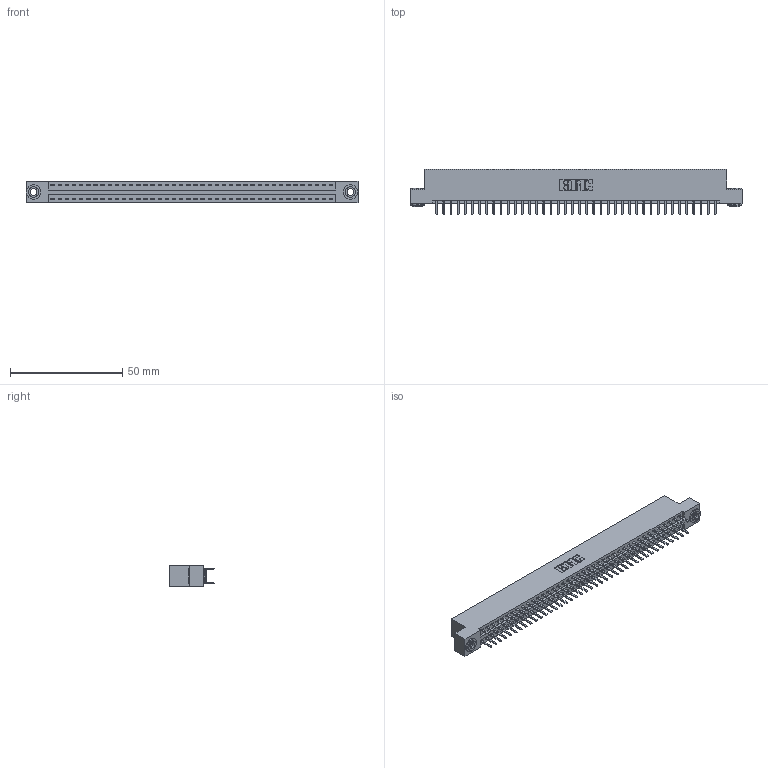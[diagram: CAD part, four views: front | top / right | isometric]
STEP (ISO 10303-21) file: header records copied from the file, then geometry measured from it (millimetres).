
FILE_DESCRIPTION (( 'STEP AP203' ), '1' );
FILE_NAME ('396-080-520-203.STEP', '2019-10-30T22:28:11', ( '' ), ( '' ), 'SwSTEP 2.0', 'SolidWorks 2016', '' );
FILE_SCHEMA (( 'CONFIG_CONTROL_DESIGN' ));
Length unit declared in the file: inch
Products named in the file (4): 396-080-520-203; 345-292-001_345-293-120; 345-250-002_345-250-002-102; 346 Part_Flush Mounting Lugs - 0.156 Dia-TH
Assembly tree (83 placements, depth 2):
  396-080-520-203
    346 Part_Flush Mounting Lugs - 0.156 Dia-TH
    345-292-001_345-293-120  x80
    345-250-002_345-250-002-102  x2
Bounding box: 147.57 x 20.02 x 9.4 mm (x, y, z)
Volume: 14359 mm3; surface area: 19837.7 mm2
Topology: 83 solids, 83 shells, 4640 faces, 13445 edges, 8746 vertices
Faces by surface type: plane 3046, cylinder 1586, cone 8
Entity records: 27138 total; most frequent: CARTESIAN_POINT 4463, ORIENTED_EDGE 4378, DIRECTION 4003, EDGE_CURVE 2189, VECTOR 1869, LINE 1869, VERTEX_POINT 1454, AXIS2_PLACEMENT_3D 1067
